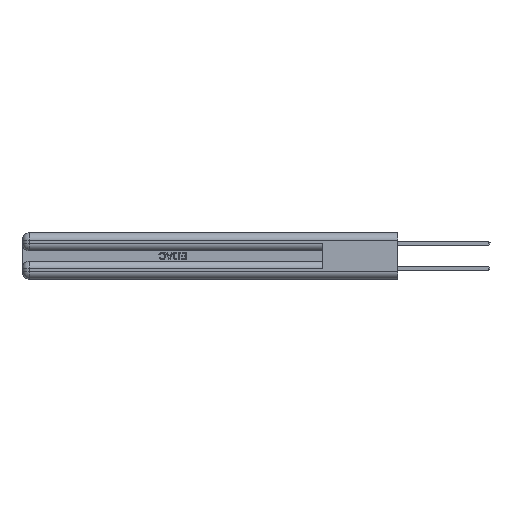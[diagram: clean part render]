
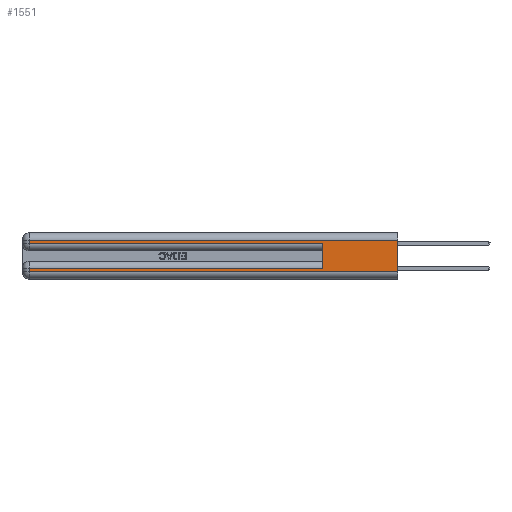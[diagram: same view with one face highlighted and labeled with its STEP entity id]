
A CAD part, left-side view. The second image highlights one B-rep face of the part: STEP entity #1551.
In plain terms, the highlighted planar face has unit normal (-1, 0, 0).
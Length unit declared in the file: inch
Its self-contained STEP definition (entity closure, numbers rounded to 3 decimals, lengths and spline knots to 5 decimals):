
#110 = LINE ( 'NONE', #43250, #18874 ) ;
#756 = VERTEX_POINT ( 'NONE', #45901 ) ;
#870 = ORIENTED_EDGE ( 'NONE', *, *, #11808, .T. ) ;
#1017 = DIRECTION ( 'NONE',  ( 0., 0., -1. ) ) ;
#1551 = ADVANCED_FACE ( 'NONE', ( #30637 ), #42376, .F. ) ;
#1673 = LINE ( 'NONE', #3200, #7384 ) ;
#2680 = CARTESIAN_POINT ( 'NONE',  ( 0., 0., 0.285 ) ) ;
#2844 = VERTEX_POINT ( 'NONE', #34443 ) ;
#2973 = DIRECTION ( 'NONE',  ( 1., 0., 0. ) ) ;
#3200 = CARTESIAN_POINT ( 'NONE',  ( 0., 2.94, 0.37 ) ) ;
#4733 = CARTESIAN_POINT ( 'NONE',  ( 0., 0.6, 0.145 ) ) ;
#5093 = LINE ( 'NONE', #2680, #23276 ) ;
#5270 = LINE ( 'NONE', #6762, #23458 ) ;
#6762 = CARTESIAN_POINT ( 'NONE',  ( 0., 0., 0.085 ) ) ;
#6885 = EDGE_CURVE ( 'NONE', #2844, #756, #5093, .T. ) ;
#7099 = DIRECTION ( 'NONE',  ( 0., 1., 0. ) ) ;
#7384 = VECTOR ( 'NONE', #13706, 39.37008 ) ;
#7385 = DIRECTION ( 'NONE',  ( 0., 1., 0. ) ) ;
#7461 = VECTOR ( 'NONE', #41424, 39.37008 ) ;
#8352 = CARTESIAN_POINT ( 'NONE',  ( 0., 0., 0.06 ) ) ;
#9460 = AXIS2_PLACEMENT_3D ( 'NONE', #24741, #2973, #42692 ) ;
#11808 = EDGE_CURVE ( 'NONE', #39791, #15798, #36496, .T. ) ;
#12472 = LINE ( 'NONE', #25564, #14183 ) ;
#12593 = EDGE_CURVE ( 'NONE', #33031, #2844, #1673, .T. ) ;
#13012 = EDGE_LOOP ( 'NONE', ( #19151, #33740, #15642, #27066, #30925, #22146, #16600, #870 ) ) ;
#13397 = EDGE_CURVE ( 'NONE', #14371, #33031, #12472, .T. ) ;
#13421 = VECTOR ( 'NONE', #44946, 39.37008 ) ;
#13706 = DIRECTION ( 'NONE',  ( 0., 0., -1. ) ) ;
#14183 = VECTOR ( 'NONE', #7385, 39.37008 ) ;
#14371 = VERTEX_POINT ( 'NONE', #19181 ) ;
#15255 = EDGE_CURVE ( 'NONE', #28763, #756, #37841, .T. ) ;
#15642 = ORIENTED_EDGE ( 'NONE', *, *, #12593, .T. ) ;
#15798 = VERTEX_POINT ( 'NONE', #44221 ) ;
#16600 = ORIENTED_EDGE ( 'NONE', *, *, #29222, .T. ) ;
#18874 = VECTOR ( 'NONE', #1017, 39.37008 ) ;
#19151 = ORIENTED_EDGE ( 'NONE', *, *, #31287, .F. ) ;
#19181 = CARTESIAN_POINT ( 'NONE',  ( 0., 0., 0.31 ) ) ;
#21556 = EDGE_CURVE ( 'NONE', #28763, #27261, #5270, .T. ) ;
#22146 = ORIENTED_EDGE ( 'NONE', *, *, #21556, .T. ) ;
#23276 = VECTOR ( 'NONE', #27961, 39.37008 ) ;
#23458 = VECTOR ( 'NONE', #7099, 39.37008 ) ;
#24448 = VECTOR ( 'NONE', #44810, 39.37008 ) ;
#24741 = CARTESIAN_POINT ( 'NONE',  ( 0., 0., 0.37 ) ) ;
#25455 = CARTESIAN_POINT ( 'NONE',  ( 0., 0.6, 0.085 ) ) ;
#25564 = CARTESIAN_POINT ( 'NONE',  ( 0., 0., 0.31 ) ) ;
#27066 = ORIENTED_EDGE ( 'NONE', *, *, #6885, .T. ) ;
#27261 = VERTEX_POINT ( 'NONE', #45231 ) ;
#27961 = DIRECTION ( 'NONE',  ( 0., -1., 0. ) ) ;
#28763 = VERTEX_POINT ( 'NONE', #25455 ) ;
#29222 = EDGE_CURVE ( 'NONE', #27261, #39791, #110, .T. ) ;
#30637 = FACE_OUTER_BOUND ( 'NONE', #13012, .T. ) ;
#30925 = ORIENTED_EDGE ( 'NONE', *, *, #15255, .F. ) ;
#31287 = EDGE_CURVE ( 'NONE', #14371, #15798, #45445, .T. ) ;
#33031 = VERTEX_POINT ( 'NONE', #46409 ) ;
#33740 = ORIENTED_EDGE ( 'NONE', *, *, #13397, .T. ) ;
#34443 = CARTESIAN_POINT ( 'NONE',  ( 0., 2.94, 0.285 ) ) ;
#36496 = LINE ( 'NONE', #8352, #7461 ) ;
#37841 = LINE ( 'NONE', #4733, #13421 ) ;
#39791 = VERTEX_POINT ( 'NONE', #46631 ) ;
#41424 = DIRECTION ( 'NONE',  ( 0., -1., 0. ) ) ;
#42376 = PLANE ( 'NONE',  #9460 ) ;
#42692 = DIRECTION ( 'NONE',  ( 0., 0., -1. ) ) ;
#43250 = CARTESIAN_POINT ( 'NONE',  ( 0., 2.94, 0.37 ) ) ;
#44221 = CARTESIAN_POINT ( 'NONE',  ( 0., 0., 0.06 ) ) ;
#44810 = DIRECTION ( 'NONE',  ( 0., 0., -1. ) ) ;
#44946 = DIRECTION ( 'NONE',  ( 0., 0., 1. ) ) ;
#45124 = CARTESIAN_POINT ( 'NONE',  ( 0., 0., 0.37 ) ) ;
#45231 = CARTESIAN_POINT ( 'NONE',  ( 0., 2.94, 0.085 ) ) ;
#45445 = LINE ( 'NONE', #45124, #24448 ) ;
#45901 = CARTESIAN_POINT ( 'NONE',  ( 0., 0.6, 0.285 ) ) ;
#46409 = CARTESIAN_POINT ( 'NONE',  ( 0., 2.94, 0.31 ) ) ;
#46631 = CARTESIAN_POINT ( 'NONE',  ( 0., 2.94, 0.06 ) ) ;
